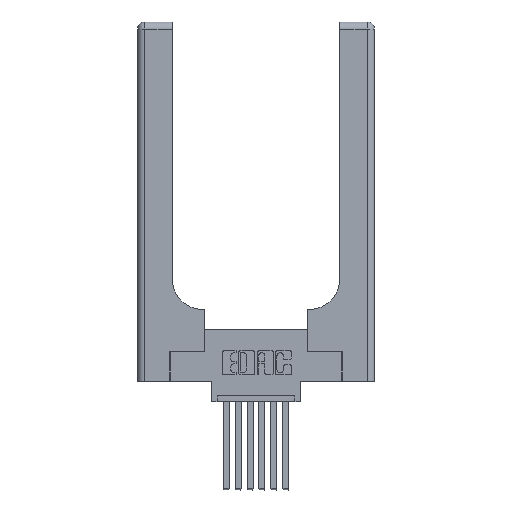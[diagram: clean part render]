
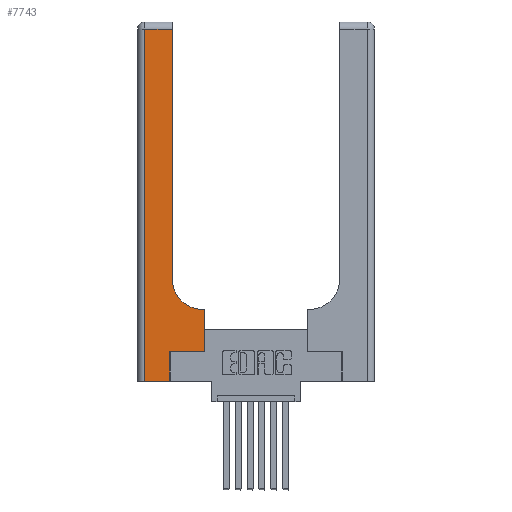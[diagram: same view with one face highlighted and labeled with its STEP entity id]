
A CAD part, top view. The second image highlights one B-rep face of the part: STEP entity #7743.
In plain terms, the highlighted planar face has unit normal (0, 0, 1).
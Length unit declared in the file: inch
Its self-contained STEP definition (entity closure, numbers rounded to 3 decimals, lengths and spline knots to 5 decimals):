
#124 = CARTESIAN_POINT ( 'NONE',  ( 0., 0., 0.37 ) ) ;
#259 = EDGE_CURVE ( 'NONE', #10010, #10228, #2759, .T. ) ;
#283 = CARTESIAN_POINT ( 'NONE',  ( 0.2915, 3., 0.37 ) ) ;
#311 = LINE ( 'NONE', #4616, #3625 ) ;
#449 = CARTESIAN_POINT ( 'NONE',  ( 0.06, 2.94, 0.37 ) ) ;
#942 = ORIENTED_EDGE ( 'NONE', *, *, #7687, .T. ) ;
#1258 = VERTEX_POINT ( 'NONE', #10436 ) ;
#1414 = VECTOR ( 'NONE', #4787, 39.37008 ) ;
#1689 = DIRECTION ( 'NONE',  ( 0., -1., 0. ) ) ;
#2017 = VECTOR ( 'NONE', #12019, 39.37008 ) ;
#2120 = LINE ( 'NONE', #124, #7914 ) ;
#2366 = LINE ( 'NONE', #3708, #2017 ) ;
#2503 = EDGE_CURVE ( 'NONE', #1258, #10010, #2366, .T. ) ;
#2593 = DIRECTION ( 'NONE',  ( 0., 1., 0. ) ) ;
#2601 = CARTESIAN_POINT ( 'NONE',  ( 0.5415, 0.85, 0.37 ) ) ;
#2707 = CARTESIAN_POINT ( 'NONE',  ( 0.269, 0., 0.37 ) ) ;
#2759 = CIRCLE ( 'NONE', #7979, 0.25 ) ;
#3011 = LINE ( 'NONE', #12716, #7764 ) ;
#3172 = CARTESIAN_POINT ( 'NONE',  ( 0.06, 0., 0.37 ) ) ;
#3552 = ORIENTED_EDGE ( 'NONE', *, *, #9094, .T. ) ;
#3606 = ORIENTED_EDGE ( 'NONE', *, *, #259, .T. ) ;
#3625 = VECTOR ( 'NONE', #10275, 39.37008 ) ;
#3708 = CARTESIAN_POINT ( 'NONE',  ( 0.2915, 0.6, 0.37 ) ) ;
#3816 = CARTESIAN_POINT ( 'NONE',  ( 0.5585, 0.25, 0.37 ) ) ;
#4084 = CARTESIAN_POINT ( 'NONE',  ( 0.5585, 0.25, 0.37 ) ) ;
#4616 = CARTESIAN_POINT ( 'NONE',  ( 0.269, 0.25, 0.37 ) ) ;
#4662 = ORIENTED_EDGE ( 'NONE', *, *, #10761, .T. ) ;
#4787 = DIRECTION ( 'NONE',  ( -1., 0., 0. ) ) ;
#5539 = CARTESIAN_POINT ( 'NONE',  ( 0.269, 0.25, 0.37 ) ) ;
#5665 = ORIENTED_EDGE ( 'NONE', *, *, #2503, .T. ) ;
#5703 = DIRECTION ( 'NONE',  ( 0., 1., 0. ) ) ;
#5825 = VECTOR ( 'NONE', #1689, 39.37008 ) ;
#5882 = DIRECTION ( 'NONE',  ( 1., 0., 0. ) ) ;
#5903 = CARTESIAN_POINT ( 'NONE',  ( 0.2915, 0.85, 0.37 ) ) ;
#5932 = DIRECTION ( 'NONE',  ( 0., 0., -1. ) ) ;
#6222 = VERTEX_POINT ( 'NONE', #13819 ) ;
#6711 = ORIENTED_EDGE ( 'NONE', *, *, #10095, .T. ) ;
#6913 = CARTESIAN_POINT ( 'NONE',  ( 0.5415, 0.6, 0.37 ) ) ;
#7050 = LINE ( 'NONE', #10215, #1414 ) ;
#7277 = VERTEX_POINT ( 'NONE', #449 ) ;
#7413 = LINE ( 'NONE', #10504, #5825 ) ;
#7609 = VECTOR ( 'NONE', #5703, 39.37008 ) ;
#7687 = EDGE_CURVE ( 'NONE', #10228, #6222, #14433, .T. ) ;
#7743 = ADVANCED_FACE ( 'NONE', ( #9512 ), #13534, .F. ) ;
#7764 = VECTOR ( 'NONE', #9722, 39.37008 ) ;
#7810 = VERTEX_POINT ( 'NONE', #2707 ) ;
#7914 = VECTOR ( 'NONE', #10317, 39.37008 ) ;
#7979 = AXIS2_PLACEMENT_3D ( 'NONE', #2601, #5932, #5882 ) ;
#8136 = ORIENTED_EDGE ( 'NONE', *, *, #9157, .T. ) ;
#8902 = EDGE_CURVE ( 'NONE', #6222, #7277, #7050, .T. ) ;
#9094 = EDGE_CURVE ( 'NONE', #7277, #10221, #7413, .T. ) ;
#9157 = EDGE_CURVE ( 'NONE', #7810, #11048, #3011, .T. ) ;
#9512 = FACE_OUTER_BOUND ( 'NONE', #11762, .T. ) ;
#9722 = DIRECTION ( 'NONE',  ( 0., 1., 0. ) ) ;
#10010 = VERTEX_POINT ( 'NONE', #6913 ) ;
#10095 = EDGE_CURVE ( 'NONE', #10221, #7810, #2120, .T. ) ;
#10215 = CARTESIAN_POINT ( 'NONE',  ( 0., 2.94, 0.37 ) ) ;
#10221 = VERTEX_POINT ( 'NONE', #3172 ) ;
#10228 = VERTEX_POINT ( 'NONE', #5903 ) ;
#10275 = DIRECTION ( 'NONE',  ( 1., 0., 0. ) ) ;
#10317 = DIRECTION ( 'NONE',  ( 1., 0., 0. ) ) ;
#10436 = CARTESIAN_POINT ( 'NONE',  ( 0.5585, 0.6, 0.37 ) ) ;
#10504 = CARTESIAN_POINT ( 'NONE',  ( 0.06, 3., 0.37 ) ) ;
#10761 = EDGE_CURVE ( 'NONE', #13212, #1258, #10855, .T. ) ;
#10855 = LINE ( 'NONE', #3816, #14378 ) ;
#11048 = VERTEX_POINT ( 'NONE', #5539 ) ;
#11297 = CARTESIAN_POINT ( 'NONE',  ( 0., 3., 0.37 ) ) ;
#11439 = DIRECTION ( 'NONE',  ( 0., 0., -1. ) ) ;
#11715 = ORIENTED_EDGE ( 'NONE', *, *, #8902, .T. ) ;
#11762 = EDGE_LOOP ( 'NONE', ( #942, #11715, #3552, #6711, #8136, #12321, #4662, #5665, #3606 ) ) ;
#12019 = DIRECTION ( 'NONE',  ( -1., 0., 0. ) ) ;
#12321 = ORIENTED_EDGE ( 'NONE', *, *, #12554, .T. ) ;
#12541 = DIRECTION ( 'NONE',  ( -1., 0., 0. ) ) ;
#12554 = EDGE_CURVE ( 'NONE', #11048, #13212, #311, .T. ) ;
#12716 = CARTESIAN_POINT ( 'NONE',  ( 0.269, 0., 0.37 ) ) ;
#13212 = VERTEX_POINT ( 'NONE', #4084 ) ;
#13534 = PLANE ( 'NONE',  #13897 ) ;
#13819 = CARTESIAN_POINT ( 'NONE',  ( 0.2915, 2.94, 0.37 ) ) ;
#13897 = AXIS2_PLACEMENT_3D ( 'NONE', #11297, #11439, #12541 ) ;
#14378 = VECTOR ( 'NONE', #2593, 39.37008 ) ;
#14433 = LINE ( 'NONE', #283, #7609 ) ;
